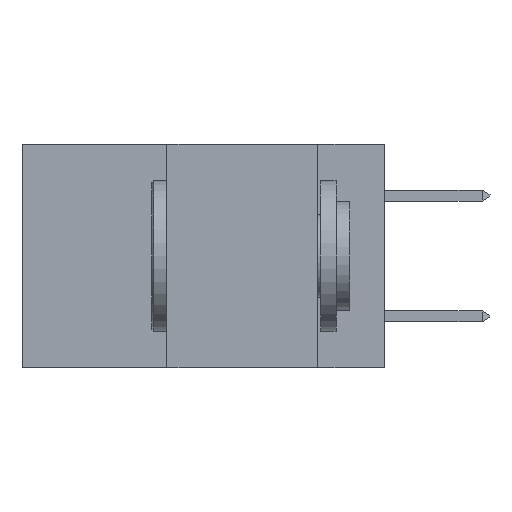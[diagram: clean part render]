
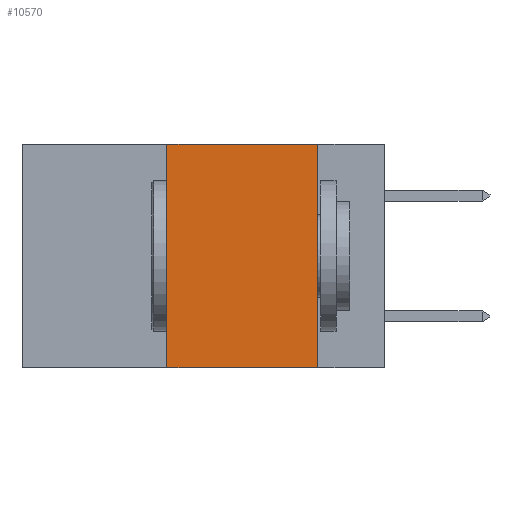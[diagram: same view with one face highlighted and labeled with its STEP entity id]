
A CAD part, left-side view. The second image highlights one B-rep face of the part: STEP entity #10570.
In plain terms, the highlighted planar face has unit normal (-1, 0, 0).
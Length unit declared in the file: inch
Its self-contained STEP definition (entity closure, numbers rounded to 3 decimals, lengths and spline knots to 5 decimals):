
#2020 = ORIENTED_EDGE ( 'NONE', *, *, #18275, .F. ) ;
#2070 = VECTOR ( 'NONE', #7823, 39.37008 ) ;
#3284 = VECTOR ( 'NONE', #6539, 39.37008 ) ;
#3586 = CARTESIAN_POINT ( 'NONE',  ( 0., 0.36, 0. ) ) ;
#3665 = LINE ( 'NONE', #3586, #23186 ) ;
#4380 = EDGE_CURVE ( 'NONE', #10589, #23117, #23691, .T. ) ;
#4836 = CARTESIAN_POINT ( 'NONE',  ( 0., 0.11, 0. ) ) ;
#5065 = DIRECTION ( 'NONE',  ( 1., 0., 0. ) ) ;
#5468 = DIRECTION ( 'NONE',  ( 0., -1., 0. ) ) ;
#6539 = DIRECTION ( 'NONE',  ( 0., 0., -1. ) ) ;
#6887 = PLANE ( 'NONE',  #22316 ) ;
#7823 = DIRECTION ( 'NONE',  ( 0., -1., 0. ) ) ;
#9328 = FACE_OUTER_BOUND ( 'NONE', #13375, .T. ) ;
#10025 = CARTESIAN_POINT ( 'NONE',  ( 0., 0.6, -0.37 ) ) ;
#10168 = VECTOR ( 'NONE', #5468, 39.37008 ) ;
#10273 = CARTESIAN_POINT ( 'NONE',  ( 0., 0.36, -0.37 ) ) ;
#10570 = ADVANCED_FACE ( 'NONE', ( #9328 ), #6887, .F. ) ;
#10589 = VERTEX_POINT ( 'NONE', #16834 ) ;
#12401 = LINE ( 'NONE', #18826, #3284 ) ;
#13066 = EDGE_CURVE ( 'NONE', #23117, #18054, #12401, .T. ) ;
#13334 = ORIENTED_EDGE ( 'NONE', *, *, #4380, .F. ) ;
#13375 = EDGE_LOOP ( 'NONE', ( #14917, #13334, #2020, #24410 ) ) ;
#14917 = ORIENTED_EDGE ( 'NONE', *, *, #13066, .F. ) ;
#14986 = LINE ( 'NONE', #10025, #2070 ) ;
#16834 = CARTESIAN_POINT ( 'NONE',  ( 0., 0.36, 0. ) ) ;
#18054 = VERTEX_POINT ( 'NONE', #21100 ) ;
#18275 = EDGE_CURVE ( 'NONE', #24474, #10589, #3665, .T. ) ;
#18416 = EDGE_CURVE ( 'NONE', #24474, #18054, #14986, .T. ) ;
#18826 = CARTESIAN_POINT ( 'NONE',  ( 0., 0.11, 0. ) ) ;
#19691 = DIRECTION ( 'NONE',  ( 0., 0., 1. ) ) ;
#20853 = CARTESIAN_POINT ( 'NONE',  ( 0., 0.6, 0. ) ) ;
#21100 = CARTESIAN_POINT ( 'NONE',  ( 0., 0.11, -0.37 ) ) ;
#22316 = AXIS2_PLACEMENT_3D ( 'NONE', #22996, #5065, #25177 ) ;
#22996 = CARTESIAN_POINT ( 'NONE',  ( 0., 0.6, 0. ) ) ;
#23117 = VERTEX_POINT ( 'NONE', #4836 ) ;
#23186 = VECTOR ( 'NONE', #19691, 39.37008 ) ;
#23691 = LINE ( 'NONE', #20853, #10168 ) ;
#24410 = ORIENTED_EDGE ( 'NONE', *, *, #18416, .T. ) ;
#24474 = VERTEX_POINT ( 'NONE', #10273 ) ;
#25177 = DIRECTION ( 'NONE',  ( 0., 0., -1. ) ) ;
